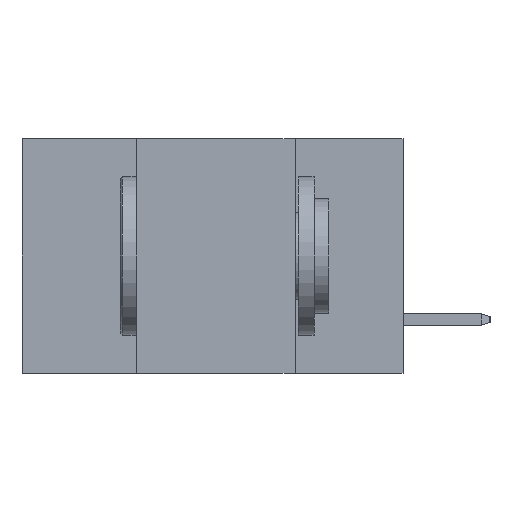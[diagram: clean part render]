
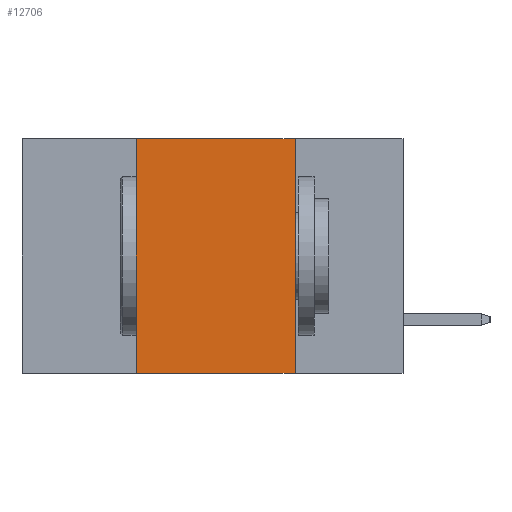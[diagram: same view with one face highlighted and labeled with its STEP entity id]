
A CAD part, left-side view. The second image highlights one B-rep face of the part: STEP entity #12706.
In plain terms, the highlighted planar face has unit normal (-1, 0, 0).
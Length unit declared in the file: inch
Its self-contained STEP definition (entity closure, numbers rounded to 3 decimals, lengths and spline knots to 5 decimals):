
#590 = EDGE_CURVE ( 'NONE', #6961, #9515, #13239, .T. ) ;
#721 = EDGE_CURVE ( 'NONE', #3691, #9515, #12498, .T. ) ;
#788 = CARTESIAN_POINT ( 'NONE',  ( 0., 0.42, -0.37 ) ) ;
#1108 = EDGE_LOOP ( 'NONE', ( #12919, #7759, #9184, #2699 ) ) ;
#1184 = DIRECTION ( 'NONE',  ( 1., 0., 0. ) ) ;
#2020 = EDGE_CURVE ( 'NONE', #4183, #6961, #3056, .T. ) ;
#2699 = ORIENTED_EDGE ( 'NONE', *, *, #721, .T. ) ;
#2883 = AXIS2_PLACEMENT_3D ( 'NONE', #13336, #1184, #14515 ) ;
#3056 = LINE ( 'NONE', #14412, #13396 ) ;
#3139 = CARTESIAN_POINT ( 'NONE',  ( 0., 0.42, 0. ) ) ;
#3691 = VERTEX_POINT ( 'NONE', #788 ) ;
#4055 = VECTOR ( 'NONE', #4341, 39.37008 ) ;
#4183 = VERTEX_POINT ( 'NONE', #10088 ) ;
#4341 = DIRECTION ( 'NONE',  ( 0., 0., 1. ) ) ;
#5086 = CARTESIAN_POINT ( 'NONE',  ( 0., 0.17, 0. ) ) ;
#5442 = CARTESIAN_POINT ( 'NONE',  ( 0., 0.6, -0.37 ) ) ;
#6229 = CARTESIAN_POINT ( 'NONE',  ( 0., 0.17, -0.37 ) ) ;
#6961 = VERTEX_POINT ( 'NONE', #7319 ) ;
#7319 = CARTESIAN_POINT ( 'NONE',  ( 0., 0.17, 0. ) ) ;
#7545 = DIRECTION ( 'NONE',  ( 0., -1., 0. ) ) ;
#7759 = ORIENTED_EDGE ( 'NONE', *, *, #2020, .F. ) ;
#8838 = PLANE ( 'NONE',  #2883 ) ;
#9184 = ORIENTED_EDGE ( 'NONE', *, *, #11773, .F. ) ;
#9515 = VERTEX_POINT ( 'NONE', #6229 ) ;
#9543 = DIRECTION ( 'NONE',  ( 0., 0., -1. ) ) ;
#9904 = DIRECTION ( 'NONE',  ( 0., -1., 0. ) ) ;
#10088 = CARTESIAN_POINT ( 'NONE',  ( 0., 0.42, 0. ) ) ;
#11101 = LINE ( 'NONE', #3139, #4055 ) ;
#11773 = EDGE_CURVE ( 'NONE', #3691, #4183, #11101, .T. ) ;
#11856 = VECTOR ( 'NONE', #9543, 39.37008 ) ;
#12498 = LINE ( 'NONE', #5442, #13030 ) ;
#12706 = ADVANCED_FACE ( 'NONE', ( #13567 ), #8838, .F. ) ;
#12919 = ORIENTED_EDGE ( 'NONE', *, *, #590, .F. ) ;
#13030 = VECTOR ( 'NONE', #9904, 39.37008 ) ;
#13239 = LINE ( 'NONE', #5086, #11856 ) ;
#13336 = CARTESIAN_POINT ( 'NONE',  ( 0., 0.6, 0. ) ) ;
#13396 = VECTOR ( 'NONE', #7545, 39.37008 ) ;
#13567 = FACE_OUTER_BOUND ( 'NONE', #1108, .T. ) ;
#14412 = CARTESIAN_POINT ( 'NONE',  ( 0., 0.6, 0. ) ) ;
#14515 = DIRECTION ( 'NONE',  ( 0., 0., -1. ) ) ;
